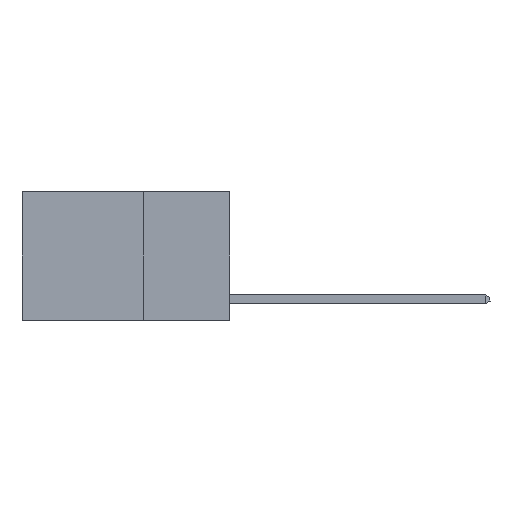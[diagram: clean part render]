
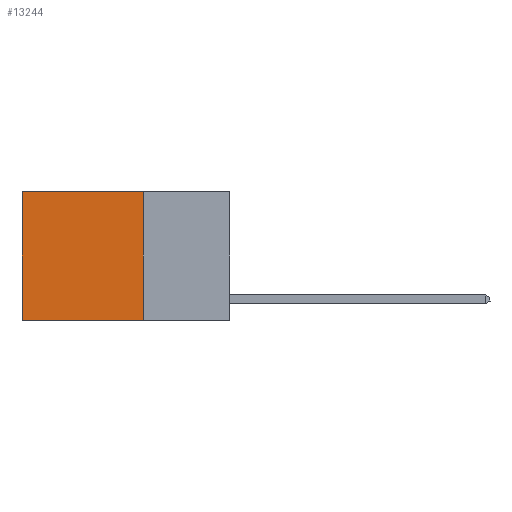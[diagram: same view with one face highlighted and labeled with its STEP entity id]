
A CAD part, left-side view. The second image highlights one B-rep face of the part: STEP entity #13244.
In plain terms, the highlighted planar face has unit normal (-1, 0, 0).
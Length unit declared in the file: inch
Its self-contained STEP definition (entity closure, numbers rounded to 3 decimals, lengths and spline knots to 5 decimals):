
#304 = DIRECTION ( 'NONE',  ( 1., 0., 0. ) ) ;
#2297 = DIRECTION ( 'NONE',  ( 0., 0., -1. ) ) ;
#2417 = EDGE_CURVE ( 'NONE', #15577, #5973, #3941, .T. ) ;
#2431 = ORIENTED_EDGE ( 'NONE', *, *, #2417, .T. ) ;
#3569 = CARTESIAN_POINT ( 'NONE',  ( 0.2625, 0.6, -0.37 ) ) ;
#3652 = LINE ( 'NONE', #18679, #14942 ) ;
#3941 = LINE ( 'NONE', #14197, #14295 ) ;
#5973 = VERTEX_POINT ( 'NONE', #11375 ) ;
#6160 = DIRECTION ( 'NONE',  ( 0., 0., -1. ) ) ;
#6948 = DIRECTION ( 'NONE',  ( 0., 0., -1. ) ) ;
#7067 = FACE_OUTER_BOUND ( 'NONE', #17721, .T. ) ;
#7396 = ORIENTED_EDGE ( 'NONE', *, *, #9215, .F. ) ;
#7633 = CARTESIAN_POINT ( 'NONE',  ( 0.2625, 0.25, 0. ) ) ;
#9008 = VERTEX_POINT ( 'NONE', #3569 ) ;
#9215 = EDGE_CURVE ( 'NONE', #15577, #13494, #16185, .T. ) ;
#9650 = CARTESIAN_POINT ( 'NONE',  ( 0.2625, 0.25, -0.37 ) ) ;
#10628 = CARTESIAN_POINT ( 'NONE',  ( 0.2625, 0.25, 0. ) ) ;
#10685 = PLANE ( 'NONE',  #12446 ) ;
#11097 = CARTESIAN_POINT ( 'NONE',  ( 0.2625, 0.6, 0. ) ) ;
#11375 = CARTESIAN_POINT ( 'NONE',  ( 0.2625, 0.6, 0. ) ) ;
#12053 = VECTOR ( 'NONE', #6948, 39.37008 ) ;
#12446 = AXIS2_PLACEMENT_3D ( 'NONE', #7633, #304, #6160 ) ;
#12784 = EDGE_CURVE ( 'NONE', #13494, #9008, #3652, .T. ) ;
#13007 = ORIENTED_EDGE ( 'NONE', *, *, #12784, .F. ) ;
#13244 = ADVANCED_FACE ( 'NONE', ( #7067 ), #10685, .F. ) ;
#13494 = VERTEX_POINT ( 'NONE', #9650 ) ;
#14197 = CARTESIAN_POINT ( 'NONE',  ( 0.2625, 0.25, 0. ) ) ;
#14236 = CARTESIAN_POINT ( 'NONE',  ( 0.2625, 0.25, 0. ) ) ;
#14295 = VECTOR ( 'NONE', #17166, 39.37008 ) ;
#14708 = EDGE_CURVE ( 'NONE', #5973, #9008, #15023, .T. ) ;
#14942 = VECTOR ( 'NONE', #18611, 39.37008 ) ;
#15023 = LINE ( 'NONE', #11097, #17326 ) ;
#15577 = VERTEX_POINT ( 'NONE', #10628 ) ;
#16185 = LINE ( 'NONE', #14236, #12053 ) ;
#16311 = ORIENTED_EDGE ( 'NONE', *, *, #14708, .T. ) ;
#17166 = DIRECTION ( 'NONE',  ( 0., 1., 0. ) ) ;
#17326 = VECTOR ( 'NONE', #2297, 39.37008 ) ;
#17721 = EDGE_LOOP ( 'NONE', ( #16311, #13007, #7396, #2431 ) ) ;
#18611 = DIRECTION ( 'NONE',  ( 0., 1., 0. ) ) ;
#18679 = CARTESIAN_POINT ( 'NONE',  ( 0.2625, 0.25, -0.37 ) ) ;
